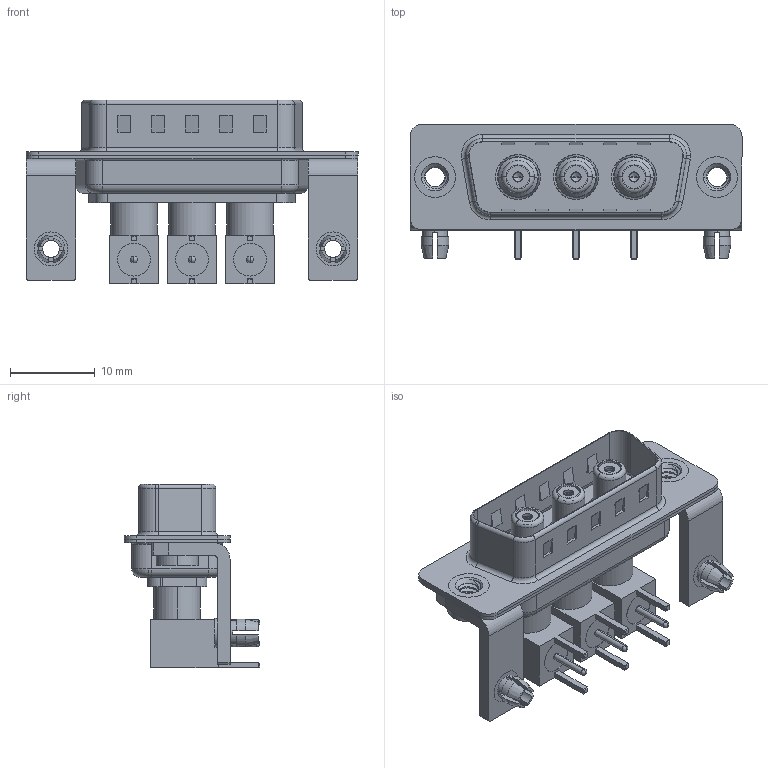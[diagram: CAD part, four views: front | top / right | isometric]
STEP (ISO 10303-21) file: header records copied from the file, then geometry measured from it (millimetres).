
FILE_DESCRIPTION (( 'STEP AP203' ), '1' );
FILE_NAME ('629-3W3-640-7TB.STEP', '2022-05-05T06:34:57', ( '' ), ( '' ), 'SwSTEP 2.0', 'SolidWorks 2020', '' );
FILE_SCHEMA (( 'CONFIG_CONTROL_DESIGN' ));
Length unit declared in the file: millimetre
Products named in the file (17): Locking Collar; 629Combo Threaded Rivet_2; Socket_RA; 629Combo Shell Rear_15 Contacts; 629Combo Board Lock; RA Back Shell; Insulator RA Pin; 629Combo Housing_3W3; Co-Ax Jack Assy_RA; 629-3W3-640-7TB; 629Combo Shell Front_15 Contacts; Co-Ax Jack_RA PC Tail; Insulator Socket; 629Combo Stabilizer Bracket; Insulator Socket 2
Assembly tree (33 placements, depth 3):
  629-3W3-640-7TB
    629Combo Housing_3W3
    629Combo Shell Rear_15 Contacts
    629Combo Shell Front_15 Contacts
    629Combo Threaded Rivet_2  x2
    629Combo Stabilizer Bracket  x2
    629Combo Board Lock  x2
    Co-Ax Jack Assy_RA
      Co-Ax Jack_RA PC Tail
      Insulator Socket
      Insulator Socket 2
      Locking Collar
      Socket_RA
      RA Back Shell
      Insulator RA Pin
    Co-Ax Jack Assy_RA
      Co-Ax Jack_RA PC Tail
      Insulator Socket
      Insulator Socket 2
      Locking Collar
      Socket_RA
      RA Back Shell
      Insulator RA Pin
    Co-Ax Jack Assy_RA
      Co-Ax Jack_RA PC Tail
      Insulator Socket
      Insulator Socket 2
      Locking Collar
      Socket_RA
      RA Back Shell
      Insulator RA Pin
Bounding box: 39.2 x 16 x 21.71 mm (x, y, z)
Volume: 3045 mm3; surface area: 8375.7 mm2
Topology: 30 solids, 30 shells, 936 faces, 2264 edges, 1421 vertices
Faces by surface type: cylinder 390, plane 378, cone 85, torus 68, bspline 9, sphere 6
Entity records: 19960 total; most frequent: CARTESIAN_POINT 4510, DIRECTION 2930, ORIENTED_EDGE 2638, EDGE_CURVE 1319, AXIS2_PLACEMENT_3D 1110, VERTEX_POINT 835, VECTOR 710, LINE 710
